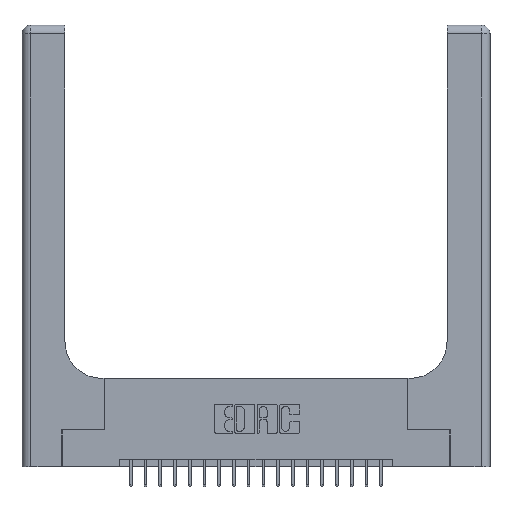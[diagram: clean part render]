
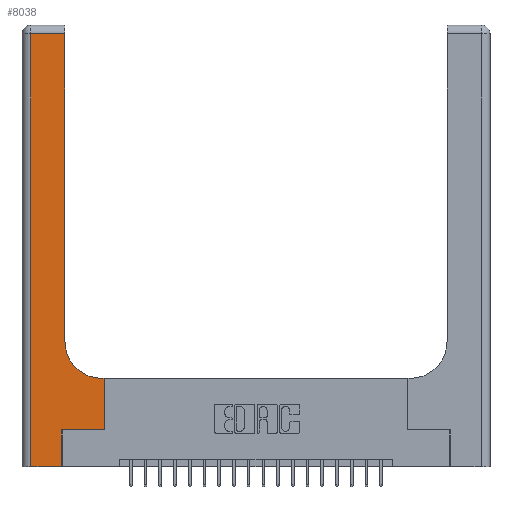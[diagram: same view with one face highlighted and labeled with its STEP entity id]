
A CAD part, top view. The second image highlights one B-rep face of the part: STEP entity #8038.
In plain terms, the highlighted planar face has unit normal (0, 0, 1).
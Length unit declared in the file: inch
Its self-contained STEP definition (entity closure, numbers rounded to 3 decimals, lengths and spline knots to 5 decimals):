
#802 = VECTOR ( 'NONE', #15962, 39.37008 ) ;
#946 = CARTESIAN_POINT ( 'NONE',  ( 0.2915, 0.6, 0.37 ) ) ;
#1120 = ORIENTED_EDGE ( 'NONE', *, *, #5272, .T. ) ;
#1401 = CARTESIAN_POINT ( 'NONE',  ( 0.06, 0., 0.37 ) ) ;
#1403 = DIRECTION ( 'NONE',  ( -1., 0., 0. ) ) ;
#1421 = EDGE_CURVE ( 'NONE', #2598, #17564, #19739, .T. ) ;
#2130 = EDGE_CURVE ( 'NONE', #17564, #19586, #17011, .T. ) ;
#2448 = DIRECTION ( 'NONE',  ( -1., 0., 0. ) ) ;
#2559 = LINE ( 'NONE', #946, #18005 ) ;
#2598 = VERTEX_POINT ( 'NONE', #18249 ) ;
#2897 = LINE ( 'NONE', #20315, #17069 ) ;
#3180 = CARTESIAN_POINT ( 'NONE',  ( 0.5415, 0.85, 0.37 ) ) ;
#3626 = LINE ( 'NONE', #4897, #5925 ) ;
#3952 = VECTOR ( 'NONE', #13335, 39.37008 ) ;
#4724 = CARTESIAN_POINT ( 'NONE',  ( 0., 2.94, 0.37 ) ) ;
#4897 = CARTESIAN_POINT ( 'NONE',  ( 0.06, 3., 0.37 ) ) ;
#5004 = CARTESIAN_POINT ( 'NONE',  ( 0.269, 0., 0.37 ) ) ;
#5272 = EDGE_CURVE ( 'NONE', #22022, #14169, #13689, .T. ) ;
#5887 = DIRECTION ( 'NONE',  ( 1., 0., 0. ) ) ;
#5925 = VECTOR ( 'NONE', #22532, 39.37008 ) ;
#6151 = CARTESIAN_POINT ( 'NONE',  ( 0.5585, 0.6, 0.37 ) ) ;
#6794 = CARTESIAN_POINT ( 'NONE',  ( 0.2915, 3., 0.37 ) ) ;
#7505 = VERTEX_POINT ( 'NONE', #15003 ) ;
#7537 = DIRECTION ( 'NONE',  ( -1., 0., 0. ) ) ;
#7731 = ORIENTED_EDGE ( 'NONE', *, *, #19731, .T. ) ;
#8038 = ADVANCED_FACE ( 'NONE', ( #16465 ), #11523, .F. ) ;
#8454 = DIRECTION ( 'NONE',  ( 1., 0., 0. ) ) ;
#8466 = CARTESIAN_POINT ( 'NONE',  ( 0.2915, 2.94, 0.37 ) ) ;
#8558 = DIRECTION ( 'NONE',  ( 0., 1., 0. ) ) ;
#8642 = VERTEX_POINT ( 'NONE', #1401 ) ;
#8675 = ORIENTED_EDGE ( 'NONE', *, *, #19251, .T. ) ;
#9578 = CARTESIAN_POINT ( 'NONE',  ( 0., 3., 0.37 ) ) ;
#9765 = EDGE_CURVE ( 'NONE', #8642, #18482, #2897, .T. ) ;
#9889 = EDGE_CURVE ( 'NONE', #11947, #7505, #17454, .T. ) ;
#10111 = ORIENTED_EDGE ( 'NONE', *, *, #9765, .T. ) ;
#11411 = DIRECTION ( 'NONE',  ( 0., 0., -1. ) ) ;
#11523 = PLANE ( 'NONE',  #14083 ) ;
#11600 = LINE ( 'NONE', #6794, #20153 ) ;
#11882 = ORIENTED_EDGE ( 'NONE', *, *, #20679, .T. ) ;
#11947 = VERTEX_POINT ( 'NONE', #8466 ) ;
#11982 = ORIENTED_EDGE ( 'NONE', *, *, #9889, .T. ) ;
#11997 = ORIENTED_EDGE ( 'NONE', *, *, #20471, .T. ) ;
#11999 = LINE ( 'NONE', #20595, #19079 ) ;
#13327 = AXIS2_PLACEMENT_3D ( 'NONE', #3180, #17166, #8454 ) ;
#13335 = DIRECTION ( 'NONE',  ( 0., 1., 0. ) ) ;
#13689 = CIRCLE ( 'NONE', #13327, 0.25 ) ;
#14083 = AXIS2_PLACEMENT_3D ( 'NONE', #9578, #11411, #7537 ) ;
#14169 = VERTEX_POINT ( 'NONE', #14573 ) ;
#14436 = CARTESIAN_POINT ( 'NONE',  ( 0.5415, 0.6, 0.37 ) ) ;
#14530 = VECTOR ( 'NONE', #1403, 39.37008 ) ;
#14573 = CARTESIAN_POINT ( 'NONE',  ( 0.2915, 0.85, 0.37 ) ) ;
#15003 = CARTESIAN_POINT ( 'NONE',  ( 0.06, 2.94, 0.37 ) ) ;
#15432 = EDGE_LOOP ( 'NONE', ( #8675, #11982, #11882, #10111, #7731, #19807, #21698, #11997, #1120 ) ) ;
#15962 = DIRECTION ( 'NONE',  ( 1., 0., 0. ) ) ;
#16465 = FACE_OUTER_BOUND ( 'NONE', #15432, .T. ) ;
#17011 = LINE ( 'NONE', #21916, #3952 ) ;
#17069 = VECTOR ( 'NONE', #5887, 39.37008 ) ;
#17166 = DIRECTION ( 'NONE',  ( 0., 0., -1. ) ) ;
#17454 = LINE ( 'NONE', #4724, #14530 ) ;
#17564 = VERTEX_POINT ( 'NONE', #19272 ) ;
#18005 = VECTOR ( 'NONE', #2448, 39.37008 ) ;
#18249 = CARTESIAN_POINT ( 'NONE',  ( 0.269, 0.25, 0.37 ) ) ;
#18482 = VERTEX_POINT ( 'NONE', #5004 ) ;
#19079 = VECTOR ( 'NONE', #8558, 39.37008 ) ;
#19251 = EDGE_CURVE ( 'NONE', #14169, #11947, #11600, .T. ) ;
#19272 = CARTESIAN_POINT ( 'NONE',  ( 0.5585, 0.25, 0.37 ) ) ;
#19586 = VERTEX_POINT ( 'NONE', #6151 ) ;
#19731 = EDGE_CURVE ( 'NONE', #18482, #2598, #11999, .T. ) ;
#19739 = LINE ( 'NONE', #19855, #802 ) ;
#19807 = ORIENTED_EDGE ( 'NONE', *, *, #1421, .T. ) ;
#19855 = CARTESIAN_POINT ( 'NONE',  ( 0.269, 0.25, 0.37 ) ) ;
#20153 = VECTOR ( 'NONE', #20649, 39.37008 ) ;
#20315 = CARTESIAN_POINT ( 'NONE',  ( 0., 0., 0.37 ) ) ;
#20471 = EDGE_CURVE ( 'NONE', #19586, #22022, #2559, .T. ) ;
#20595 = CARTESIAN_POINT ( 'NONE',  ( 0.269, 0., 0.37 ) ) ;
#20649 = DIRECTION ( 'NONE',  ( 0., 1., 0. ) ) ;
#20679 = EDGE_CURVE ( 'NONE', #7505, #8642, #3626, .T. ) ;
#21698 = ORIENTED_EDGE ( 'NONE', *, *, #2130, .T. ) ;
#21916 = CARTESIAN_POINT ( 'NONE',  ( 0.5585, 0.25, 0.37 ) ) ;
#22022 = VERTEX_POINT ( 'NONE', #14436 ) ;
#22532 = DIRECTION ( 'NONE',  ( 0., -1., 0. ) ) ;
